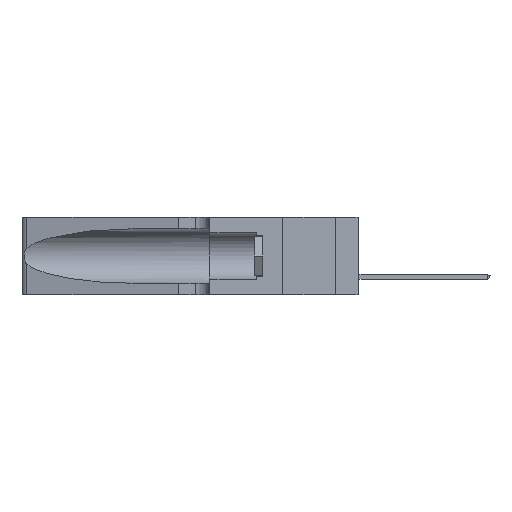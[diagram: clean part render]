
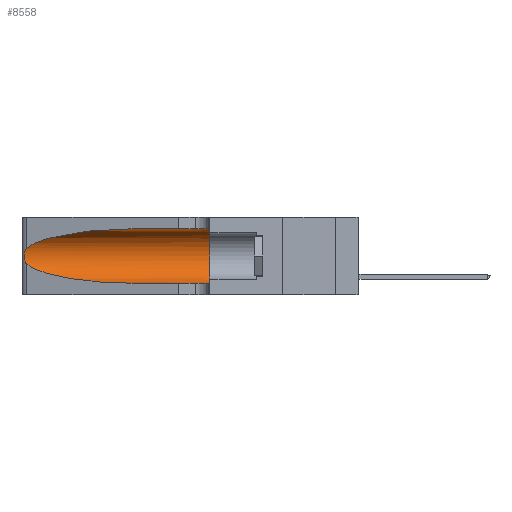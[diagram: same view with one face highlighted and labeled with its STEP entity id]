
A CAD part, left-side view. The second image highlights one B-rep face of the part: STEP entity #8558.
In plain terms, the highlighted cylindrical face has radius 3.308 mm (diameter 6.617 mm), a partial arc.
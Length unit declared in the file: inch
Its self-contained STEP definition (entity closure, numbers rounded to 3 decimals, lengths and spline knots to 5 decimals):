
#136 = AXIS2_PLACEMENT_3D ( 'NONE', #31252, #584, #23636 ) ;
#270 = EDGE_CURVE ( 'NONE', #7030, #21985, #13327, .T. ) ;
#584 = DIRECTION ( 'NONE',  ( 0., -1., 0. ) ) ;
#1643 = CARTESIAN_POINT ( 'NONE',  ( 0.25487, 1.22718, 0.14631 ) ) ;
#1716 =( BOUNDED_CURVE ( )  B_SPLINE_CURVE ( 3, ( #4176, #32081, #6943, #31753 ),
 .UNSPECIFIED., .F., .T. ) 
 B_SPLINE_CURVE_WITH_KNOTS ( ( 4, 4 ),
 ( 1.5708, 2.84003 ),
 .UNSPECIFIED. ) 
 CURVE ( )  GEOMETRIC_REPRESENTATION_ITEM ( )  RATIONAL_B_SPLINE_CURVE ( ( 1., 0.87, 0.87, 1. ) ) 
 REPRESENTATION_ITEM ( '' )  );
#3103 = VERTEX_POINT ( 'NONE', #28353 ) ;
#3535 = CARTESIAN_POINT ( 'NONE',  ( 0.1305, 0.72297, 0.31525 ) ) ;
#4030 = CARTESIAN_POINT ( 'NONE',  ( 0.2373, 1.15595, 0.08982 ) ) ;
#4176 = CARTESIAN_POINT ( 'NONE',  ( 0.1305, 0.72297, 0.31525 ) ) ;
#4977 = ORIENTED_EDGE ( 'NONE', *, *, #5090, .T. ) ;
#5090 = EDGE_CURVE ( 'NONE', #27679, #14378, #24181, .T. ) ;
#5423 = CARTESIAN_POINT ( 'NONE',  ( 0.25787, 1.23484, 0.2124 ) ) ;
#5527 = ORIENTED_EDGE ( 'NONE', *, *, #17666, .T. ) ;
#6306 = EDGE_CURVE ( 'NONE', #18708, #7030, #7646, .T. ) ;
#6943 = CARTESIAN_POINT ( 'NONE',  ( 0.2373, 1.15595, 0.28018 ) ) ;
#6965 = CARTESIAN_POINT ( 'NONE',  ( 0.1305, 0.35, 0.31525 ) ) ;
#7030 = VERTEX_POINT ( 'NONE', #6965 ) ;
#7646 = LINE ( 'NONE', #19103, #24618 ) ;
#7889 = CARTESIAN_POINT ( 'NONE',  ( 0.25487, 1.22718, 0.22369 ) ) ;
#8001 = CARTESIAN_POINT ( 'NONE',  ( 0.25854, 1.2359, 0.20912 ) ) ;
#8558 = ADVANCED_FACE ( 'NONE', ( #31187 ), #16617, .F. ) ;
#9173 = DIRECTION ( 'NONE',  ( 0., -1., 0. ) ) ;
#9242 = CARTESIAN_POINT ( 'NONE',  ( 0.26017, 1.23833, 0.17102 ) ) ;
#10414 = CARTESIAN_POINT ( 'NONE',  ( 0.25639, 1.23184, 0.21858 ) ) ;
#11114 = CARTESIAN_POINT ( 'NONE',  ( 0.1305, 0.35, 0.185 ) ) ;
#11704 = CARTESIAN_POINT ( 'NONE',  ( 0.25789, 1.23486, 0.15765 ) ) ;
#12624 = CARTESIAN_POINT ( 'NONE',  ( 0.25555, 1.22993, 0.14849 ) ) ;
#13327 = CIRCLE ( 'NONE', #20480, 0.13025 ) ;
#13944 = DIRECTION ( 'NONE',  ( 0., -1., 0. ) ) ;
#14124 = CARTESIAN_POINT ( 'NONE',  ( 0.25856, 1.23593, 0.16098 ) ) ;
#14378 = VERTEX_POINT ( 'NONE', #1643 ) ;
#15637 = ORIENTED_EDGE ( 'NONE', *, *, #16850, .T. ) ;
#15913 = EDGE_CURVE ( 'NONE', #18708, #27679, #1716, .T. ) ;
#16551 = VECTOR ( 'NONE', #9173, 39.37008 ) ;
#16617 = CYLINDRICAL_SURFACE ( 'NONE', #136, 0.13025 ) ;
#16850 = EDGE_CURVE ( 'NONE', #3103, #21985, #29954, .T. ) ;
#17666 = EDGE_CURVE ( 'NONE', #14378, #3103, #30577, .T. ) ;
#17823 = CARTESIAN_POINT ( 'NONE',  ( 0.25487, 1.22718, 0.14631 ) ) ;
#18025 = CARTESIAN_POINT ( 'NONE',  ( 0.1305, 0.35, 0.05475 ) ) ;
#18708 = VERTEX_POINT ( 'NONE', #3535 ) ;
#19103 = CARTESIAN_POINT ( 'NONE',  ( 0.1305, 1.61858, 0.31525 ) ) ;
#19128 = CARTESIAN_POINT ( 'NONE',  ( 0.25487, 1.22718, 0.14631 ) ) ;
#19623 = ORIENTED_EDGE ( 'NONE', *, *, #15913, .T. ) ;
#20480 = AXIS2_PLACEMENT_3D ( 'NONE', #11114, #28612, #23326 ) ;
#20677 = CARTESIAN_POINT ( 'NONE',  ( 0.26018, 1.23835, 0.19895 ) ) ;
#21656 = CARTESIAN_POINT ( 'NONE',  ( 0.18966, 0.96281, 0.05475 ) ) ;
#21985 = VERTEX_POINT ( 'NONE', #18025 ) ;
#22060 = ORIENTED_EDGE ( 'NONE', *, *, #6306, .F. ) ;
#23209 = CARTESIAN_POINT ( 'NONE',  ( 0.26075, 1.23896, 0.19203 ) ) ;
#23326 = DIRECTION ( 'NONE',  ( 0., 0., 1. ) ) ;
#23636 = DIRECTION ( 'NONE',  ( 0., 0., -1. ) ) ;
#24181 = B_SPLINE_CURVE_WITH_KNOTS ( 'NONE', 3,
 ( #7889, #25507, #10414, #5423, #8001, #20677, #23209, #26637, #9242, #14124, #11704, #31842, #12624, #17823 ),
 .UNSPECIFIED., .F., .F.,
 ( 4, 2, 2, 2, 2, 2, 4 ),
 ( 0., 0.00027, 0.00053, 0.00107, 0.0016, 0.00187, 0.00214 ),
 .UNSPECIFIED. ) ;
#24618 = VECTOR ( 'NONE', #13944, 39.37008 ) ;
#25507 = CARTESIAN_POINT ( 'NONE',  ( 0.25555, 1.22994, 0.2215 ) ) ;
#25712 = CARTESIAN_POINT ( 'NONE',  ( 0.25487, 1.22718, 0.22369 ) ) ;
#26637 = CARTESIAN_POINT ( 'NONE',  ( 0.26075, 1.23896, 0.178 ) ) ;
#27029 = CARTESIAN_POINT ( 'NONE',  ( 0.1305, 1.61858, 0.05475 ) ) ;
#27679 = VERTEX_POINT ( 'NONE', #25712 ) ;
#28353 = CARTESIAN_POINT ( 'NONE',  ( 0.1305, 0.72297, 0.05475 ) ) ;
#28612 = DIRECTION ( 'NONE',  ( 0., 1., 0. ) ) ;
#28898 = CARTESIAN_POINT ( 'NONE',  ( 0.1305, 0.72297, 0.05475 ) ) ;
#29954 = LINE ( 'NONE', #27029, #16551 ) ;
#30577 =( BOUNDED_CURVE ( )  B_SPLINE_CURVE ( 3, ( #19128, #4030, #21656, #28898 ),
 .UNSPECIFIED., .F., .F. ) 
 B_SPLINE_CURVE_WITH_KNOTS ( ( 4, 4 ),
 ( 3.44316, 4.71239 ),
 .UNSPECIFIED. ) 
 CURVE ( )  GEOMETRIC_REPRESENTATION_ITEM ( )  RATIONAL_B_SPLINE_CURVE ( ( 1., 0.87, 0.87, 1. ) ) 
 REPRESENTATION_ITEM ( '' )  );
#30725 = EDGE_LOOP ( 'NONE', ( #19623, #4977, #5527, #15637, #32516, #22060 ) ) ;
#31187 = FACE_OUTER_BOUND ( 'NONE', #30725, .T. ) ;
#31252 = CARTESIAN_POINT ( 'NONE',  ( 0.1305, 1.61858, 0.185 ) ) ;
#31753 = CARTESIAN_POINT ( 'NONE',  ( 0.25487, 1.22718, 0.22369 ) ) ;
#31842 = CARTESIAN_POINT ( 'NONE',  ( 0.25639, 1.23186, 0.15144 ) ) ;
#32081 = CARTESIAN_POINT ( 'NONE',  ( 0.18966, 0.96281, 0.31525 ) ) ;
#32516 = ORIENTED_EDGE ( 'NONE', *, *, #270, .F. ) ;
